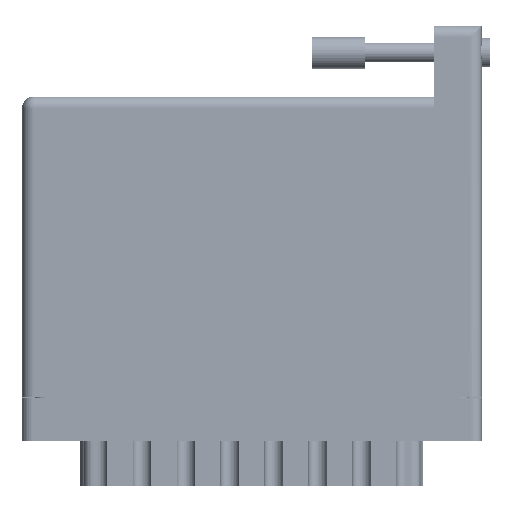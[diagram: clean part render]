
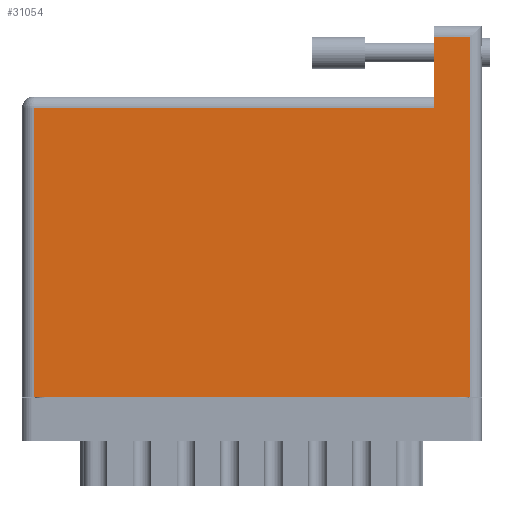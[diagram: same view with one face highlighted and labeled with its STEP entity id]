
A CAD part, front view. The second image highlights one B-rep face of the part: STEP entity #31054.
In plain terms, the highlighted face is planar.
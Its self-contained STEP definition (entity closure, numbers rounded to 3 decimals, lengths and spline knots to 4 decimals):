
#7037 = VECTOR ( 'NONE', #62114, 39.3701 ) ;
#7812 = CARTESIAN_POINT ( 'NONE',  ( 0., 1.775, 0. ) ) ;
#9523 = ORIENTED_EDGE ( 'NONE', *, *, #45802, .T. ) ;
#10732 = DIRECTION ( 'NONE',  ( 0., -1., 0. ) ) ;
#13931 = CARTESIAN_POINT ( 'NONE',  ( 0.07, 1.705, 0. ) ) ;
#16001 = VERTEX_POINT ( 'NONE', #13931 ) ;
#16019 = CARTESIAN_POINT ( 'NONE',  ( 2.648, 2.195, 0. ) ) ;
#16050 = CARTESIAN_POINT ( 'NONE',  ( 0.07, 0., 0. ) ) ;
#17106 = LINE ( 'NONE', #50553, #7037 ) ;
#18641 = VECTOR ( 'NONE', #20353, 39.3701 ) ;
#19960 = LINE ( 'NONE', #75134, #29189 ) ;
#20353 = DIRECTION ( 'NONE',  ( -1., 0., 0. ) ) ;
#24285 = ORIENTED_EDGE ( 'NONE', *, *, #35774, .T. ) ;
#29189 = VECTOR ( 'NONE', #10732, 39.3701 ) ;
#30221 = EDGE_CURVE ( 'NONE', #33947, #54067, #35923, .T. ) ;
#30880 = ORIENTED_EDGE ( 'NONE', *, *, #64417, .T. ) ;
#31054 = ADVANCED_FACE ( 'NONE', ( #69911 ), #56003, .F. ) ;
#32404 = EDGE_CURVE ( 'NONE', #63610, #53258, #17106, .T. ) ;
#33947 = VERTEX_POINT ( 'NONE', #65180 ) ;
#35774 = EDGE_CURVE ( 'NONE', #53258, #33947, #39859, .T. ) ;
#35923 = LINE ( 'NONE', #51500, #48861 ) ;
#36639 = ORIENTED_EDGE ( 'NONE', *, *, #61156, .T. ) ;
#39859 = LINE ( 'NONE', #16019, #43558 ) ;
#40719 = EDGE_LOOP ( 'NONE', ( #30880, #9523, #64294, #24285, #46915, #36639 ) ) ;
#42402 = CARTESIAN_POINT ( 'NONE',  ( 2.438, 2.125, 0. ) ) ;
#43558 = VECTOR ( 'NONE', #51902, 39.3701 ) ;
#43858 = DIRECTION ( 'NONE',  ( 0., 0., -1. ) ) ;
#44334 = CARTESIAN_POINT ( 'NONE',  ( 0., 1.705, 0. ) ) ;
#45687 = VERTEX_POINT ( 'NONE', #58434 ) ;
#45802 = EDGE_CURVE ( 'NONE', #16001, #63610, #47392, .T. ) ;
#46036 = DIRECTION ( 'NONE',  ( -1., 0., 0. ) ) ;
#46337 = LINE ( 'NONE', #44334, #18641 ) ;
#46915 = ORIENTED_EDGE ( 'NONE', *, *, #30221, .T. ) ;
#47392 = LINE ( 'NONE', #65336, #60270 ) ;
#48861 = VECTOR ( 'NONE', #46036, 39.3701 ) ;
#50553 = CARTESIAN_POINT ( 'NONE',  ( 0., 0., 0. ) ) ;
#51500 = CARTESIAN_POINT ( 'NONE',  ( 0., 2.125, 0. ) ) ;
#51902 = DIRECTION ( 'NONE',  ( 0., 1., 0. ) ) ;
#53258 = VERTEX_POINT ( 'NONE', #59763 ) ;
#53801 = DIRECTION ( 'NONE',  ( 0., -1., 0. ) ) ;
#54067 = VERTEX_POINT ( 'NONE', #42402 ) ;
#56003 = PLANE ( 'NONE',  #72493 ) ;
#58434 = CARTESIAN_POINT ( 'NONE',  ( 2.438, 1.705, 0. ) ) ;
#59763 = CARTESIAN_POINT ( 'NONE',  ( 2.648, 0., 0. ) ) ;
#60270 = VECTOR ( 'NONE', #53801, 39.3701 ) ;
#61156 = EDGE_CURVE ( 'NONE', #54067, #45687, #19960, .T. ) ;
#62114 = DIRECTION ( 'NONE',  ( 1., 0., 0. ) ) ;
#63610 = VERTEX_POINT ( 'NONE', #16050 ) ;
#64294 = ORIENTED_EDGE ( 'NONE', *, *, #32404, .T. ) ;
#64417 = EDGE_CURVE ( 'NONE', #45687, #16001, #46337, .T. ) ;
#65180 = CARTESIAN_POINT ( 'NONE',  ( 2.648, 2.125, 0. ) ) ;
#65336 = CARTESIAN_POINT ( 'NONE',  ( 0.07, 0., 0. ) ) ;
#69911 = FACE_OUTER_BOUND ( 'NONE', #40719, .T. ) ;
#72493 = AXIS2_PLACEMENT_3D ( 'NONE', #7812, #43858, #73455 ) ;
#73455 = DIRECTION ( 'NONE',  ( -1., 0., 0. ) ) ;
#75134 = CARTESIAN_POINT ( 'NONE',  ( 2.438, 2.195, 0. ) ) ;
